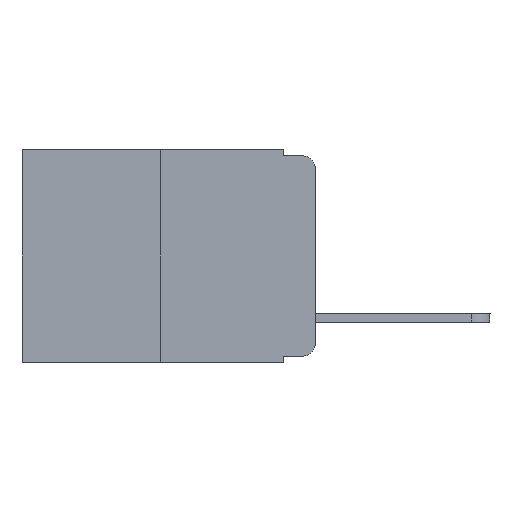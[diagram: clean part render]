
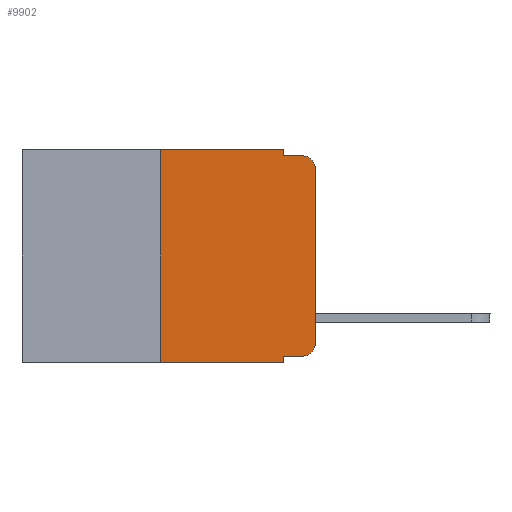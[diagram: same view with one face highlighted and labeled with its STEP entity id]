
A CAD part, left-side view. The second image highlights one B-rep face of the part: STEP entity #9902.
In plain terms, the highlighted planar face has unit normal (-1, 0, 0).
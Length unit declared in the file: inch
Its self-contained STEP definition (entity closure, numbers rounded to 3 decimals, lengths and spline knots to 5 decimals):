
#61 = VECTOR ( 'NONE', #72, 39.37008 ) ;
#72 = DIRECTION ( 'NONE',  ( 0., -1., 0. ) ) ;
#476 = VECTOR ( 'NONE', #4185, 39.37008 ) ;
#866 = VECTOR ( 'NONE', #4651, 39.37008 ) ;
#913 = VERTEX_POINT ( 'NONE', #14637 ) ;
#1226 = CARTESIAN_POINT ( 'NONE',  ( 0., 0.051, -0.333 ) ) ;
#1229 = EDGE_CURVE ( 'NONE', #15081, #14641, #2626, .T. ) ;
#1828 = CARTESIAN_POINT ( 'NONE',  ( 0., 0.051, -0.343 ) ) ;
#2098 = ORIENTED_EDGE ( 'NONE', *, *, #8680, .F. ) ;
#2134 = EDGE_CURVE ( 'NONE', #14641, #12399, #9889, .T. ) ;
#2243 = ORIENTED_EDGE ( 'NONE', *, *, #10775, .T. ) ;
#2381 = CARTESIAN_POINT ( 'NONE',  ( 0., 0.051, 0. ) ) ;
#2567 = DIRECTION ( 'NONE',  ( 0., 0., 1. ) ) ;
#2626 = LINE ( 'NONE', #10273, #476 ) ;
#2660 = FACE_OUTER_BOUND ( 'NONE', #10278, .T. ) ;
#2946 = EDGE_CURVE ( 'NONE', #12925, #3644, #5142, .T. ) ;
#3101 = ORIENTED_EDGE ( 'NONE', *, *, #10624, .T. ) ;
#3300 = VECTOR ( 'NONE', #4770, 39.37008 ) ;
#3627 = ORIENTED_EDGE ( 'NONE', *, *, #2134, .T. ) ;
#3644 = VERTEX_POINT ( 'NONE', #2381 ) ;
#3834 = ORIENTED_EDGE ( 'NONE', *, *, #1229, .T. ) ;
#3904 = LINE ( 'NONE', #13360, #11555 ) ;
#4169 = ORIENTED_EDGE ( 'NONE', *, *, #2946, .F. ) ;
#4185 = DIRECTION ( 'NONE',  ( 0., 0., 1. ) ) ;
#4221 = CARTESIAN_POINT ( 'NONE',  ( 0., 0.02, -0.03 ) ) ;
#4317 = AXIS2_PLACEMENT_3D ( 'NONE', #8989, #7482, #14096 ) ;
#4651 = DIRECTION ( 'NONE',  ( 0., 0., -1. ) ) ;
#4668 = AXIS2_PLACEMENT_3D ( 'NONE', #14157, #10380, #7793 ) ;
#4770 = DIRECTION ( 'NONE',  ( 0., -1., 0. ) ) ;
#4808 = LINE ( 'NONE', #16407, #11060 ) ;
#4970 = LINE ( 'NONE', #15371, #16142 ) ;
#5034 = LINE ( 'NONE', #11162, #3300 ) ;
#5142 = LINE ( 'NONE', #11607, #9652 ) ;
#5734 = ORIENTED_EDGE ( 'NONE', *, *, #12256, .F. ) ;
#6455 = CARTESIAN_POINT ( 'NONE',  ( 0., 0., -0.313 ) ) ;
#6565 = CARTESIAN_POINT ( 'NONE',  ( 0., 0., -0.03 ) ) ;
#6636 = LINE ( 'NONE', #10491, #61 ) ;
#6660 = VERTEX_POINT ( 'NONE', #1226 ) ;
#6665 = ORIENTED_EDGE ( 'NONE', *, *, #15801, .F. ) ;
#6737 = CIRCLE ( 'NONE', #4317, 0.02 ) ;
#7482 = DIRECTION ( 'NONE',  ( -1., 0., 0. ) ) ;
#7487 = AXIS2_PLACEMENT_3D ( 'NONE', #4221, #10617, #9354 ) ;
#7712 = CARTESIAN_POINT ( 'NONE',  ( 0., 0.02, -0.333 ) ) ;
#7747 = VERTEX_POINT ( 'NONE', #8147 ) ;
#7793 = DIRECTION ( 'NONE',  ( 0., 0., -1. ) ) ;
#8147 = CARTESIAN_POINT ( 'NONE',  ( 0., 0.051, -0.01 ) ) ;
#8680 = EDGE_CURVE ( 'NONE', #913, #12925, #3904, .T. ) ;
#8989 = CARTESIAN_POINT ( 'NONE',  ( 0., 0.02, -0.313 ) ) ;
#8997 = DIRECTION ( 'NONE',  ( 0., -1., 0. ) ) ;
#9354 = DIRECTION ( 'NONE',  ( 0., 0., -1. ) ) ;
#9402 = ORIENTED_EDGE ( 'NONE', *, *, #15956, .F. ) ;
#9652 = VECTOR ( 'NONE', #8997, 39.37008 ) ;
#9889 = CIRCLE ( 'NONE', #7487, 0.02 ) ;
#9902 = ADVANCED_FACE ( 'NONE', ( #2660 ), #12993, .F. ) ;
#10088 = ORIENTED_EDGE ( 'NONE', *, *, #13392, .T. ) ;
#10100 = DIRECTION ( 'NONE',  ( 0., 0., -1. ) ) ;
#10273 = CARTESIAN_POINT ( 'NONE',  ( 0., 0., 0. ) ) ;
#10278 = EDGE_LOOP ( 'NONE', ( #3834, #3627, #5734, #6665, #4169, #2098, #3101, #9402, #2243, #10088 ) ) ;
#10380 = DIRECTION ( 'NONE',  ( 1., 0., 0. ) ) ;
#10386 = CARTESIAN_POINT ( 'NONE',  ( 0., 0.02, -0.01 ) ) ;
#10491 = CARTESIAN_POINT ( 'NONE',  ( 0., 0.051, -0.333 ) ) ;
#10617 = DIRECTION ( 'NONE',  ( -1., 0., 0. ) ) ;
#10624 = EDGE_CURVE ( 'NONE', #913, #13660, #4970, .T. ) ;
#10775 = EDGE_CURVE ( 'NONE', #6660, #13754, #6636, .T. ) ;
#11034 = LINE ( 'NONE', #16156, #866 ) ;
#11060 = VECTOR ( 'NONE', #10100, 39.37008 ) ;
#11162 = CARTESIAN_POINT ( 'NONE',  ( 0., 0.051, -0.01 ) ) ;
#11555 = VECTOR ( 'NONE', #2567, 39.37008 ) ;
#11607 = CARTESIAN_POINT ( 'NONE',  ( 0., 0.473, 0. ) ) ;
#11797 = CARTESIAN_POINT ( 'NONE',  ( 0., 0.25, 0. ) ) ;
#12256 = EDGE_CURVE ( 'NONE', #7747, #12399, #5034, .T. ) ;
#12399 = VERTEX_POINT ( 'NONE', #10386 ) ;
#12925 = VERTEX_POINT ( 'NONE', #11797 ) ;
#12993 = PLANE ( 'NONE',  #4668 ) ;
#13360 = CARTESIAN_POINT ( 'NONE',  ( 0., 0.25, 0. ) ) ;
#13392 = EDGE_CURVE ( 'NONE', #13754, #15081, #6737, .T. ) ;
#13660 = VERTEX_POINT ( 'NONE', #1828 ) ;
#13754 = VERTEX_POINT ( 'NONE', #7712 ) ;
#13943 = DIRECTION ( 'NONE',  ( 0., -1., 0. ) ) ;
#14096 = DIRECTION ( 'NONE',  ( 0., 0., -1. ) ) ;
#14157 = CARTESIAN_POINT ( 'NONE',  ( 0., 0.473, 0. ) ) ;
#14637 = CARTESIAN_POINT ( 'NONE',  ( 0., 0.25, -0.343 ) ) ;
#14641 = VERTEX_POINT ( 'NONE', #6565 ) ;
#15081 = VERTEX_POINT ( 'NONE', #6455 ) ;
#15371 = CARTESIAN_POINT ( 'NONE',  ( 0., 0.473, -0.343 ) ) ;
#15801 = EDGE_CURVE ( 'NONE', #3644, #7747, #11034, .T. ) ;
#15956 = EDGE_CURVE ( 'NONE', #6660, #13660, #4808, .T. ) ;
#16142 = VECTOR ( 'NONE', #13943, 39.37008 ) ;
#16156 = CARTESIAN_POINT ( 'NONE',  ( 0., 0.051, 0. ) ) ;
#16407 = CARTESIAN_POINT ( 'NONE',  ( 0., 0.051, 0. ) ) ;
